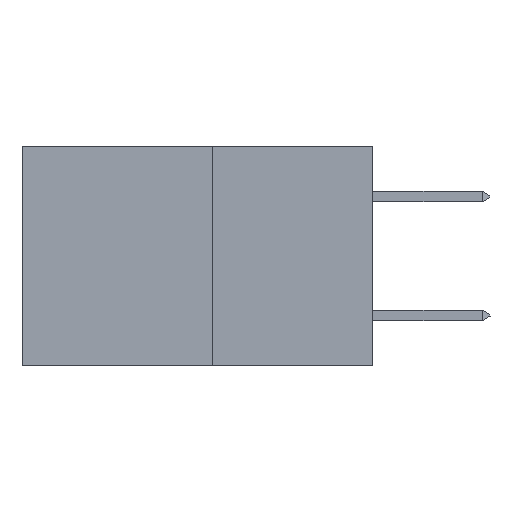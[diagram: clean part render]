
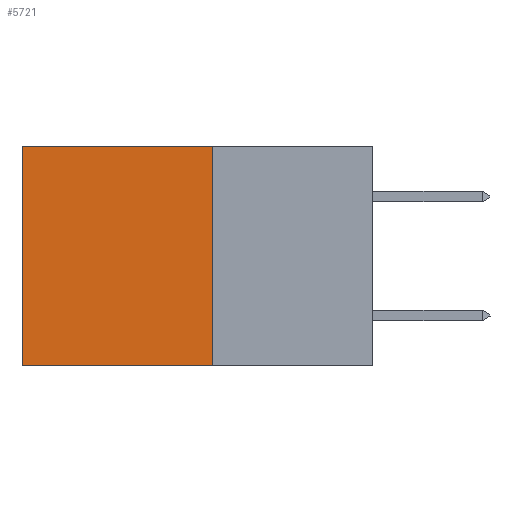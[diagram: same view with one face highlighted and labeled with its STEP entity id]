
A CAD part, left-side view. The second image highlights one B-rep face of the part: STEP entity #5721.
In plain terms, the highlighted planar face has unit normal (-1, 0, 0).
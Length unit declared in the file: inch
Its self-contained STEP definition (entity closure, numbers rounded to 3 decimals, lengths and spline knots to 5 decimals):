
#82 = AXIS2_PLACEMENT_3D ( 'NONE', #2713, #2704, #2680 ) ;
#160 = CARTESIAN_POINT ( 'NONE',  ( 0.277, 0.27, -0.37 ) ) ;
#296 = CARTESIAN_POINT ( 'NONE',  ( 0.277, 0.59, -0.37 ) ) ;
#460 = CARTESIAN_POINT ( 'NONE',  ( 0.277, 0.27, 0. ) ) ;
#487 = DIRECTION ( 'NONE',  ( 0., 1., 0. ) ) ;
#781 = EDGE_CURVE ( 'NONE', #8859, #3221, #3631, .T. ) ;
#1024 = DIRECTION ( 'NONE',  ( 0., 0., -1. ) ) ;
#1095 = VERTEX_POINT ( 'NONE', #5561 ) ;
#1116 = CARTESIAN_POINT ( 'NONE',  ( 0.277, 0.59, -0.37 ) ) ;
#2073 = LINE ( 'NONE', #460, #3802 ) ;
#2413 = CARTESIAN_POINT ( 'NONE',  ( 0.277, 0.27, -0.37 ) ) ;
#2680 = DIRECTION ( 'NONE',  ( 0., 0., -1. ) ) ;
#2704 = DIRECTION ( 'NONE',  ( 1., 0., 0. ) ) ;
#2713 = CARTESIAN_POINT ( 'NONE',  ( 0.277, 0.27, -0.37 ) ) ;
#2767 = PLANE ( 'NONE',  #82 ) ;
#3221 = VERTEX_POINT ( 'NONE', #2413 ) ;
#3456 = EDGE_CURVE ( 'NONE', #8859, #1095, #2073, .T. ) ;
#3483 = EDGE_CURVE ( 'NONE', #3221, #6343, #7754, .T. ) ;
#3631 = LINE ( 'NONE', #7511, #7600 ) ;
#3650 = ORIENTED_EDGE ( 'NONE', *, *, #3456, .T. ) ;
#3802 = VECTOR ( 'NONE', #7028, 39.37008 ) ;
#4950 = DIRECTION ( 'NONE',  ( 0., 0., -1. ) ) ;
#5561 = CARTESIAN_POINT ( 'NONE',  ( 0.277, 0.59, 0. ) ) ;
#5577 = EDGE_LOOP ( 'NONE', ( #9260, #6430, #9116, #3650 ) ) ;
#5721 = ADVANCED_FACE ( 'NONE', ( #6285 ), #2767, .F. ) ;
#5869 = VECTOR ( 'NONE', #487, 39.37008 ) ;
#6285 = FACE_OUTER_BOUND ( 'NONE', #5577, .T. ) ;
#6343 = VERTEX_POINT ( 'NONE', #296 ) ;
#6430 = ORIENTED_EDGE ( 'NONE', *, *, #3483, .F. ) ;
#7028 = DIRECTION ( 'NONE',  ( 0., 1., 0. ) ) ;
#7395 = EDGE_CURVE ( 'NONE', #1095, #6343, #7711, .T. ) ;
#7509 = VECTOR ( 'NONE', #1024, 39.37008 ) ;
#7511 = CARTESIAN_POINT ( 'NONE',  ( 0.277, 0.27, -0.37 ) ) ;
#7600 = VECTOR ( 'NONE', #4950, 39.37008 ) ;
#7711 = LINE ( 'NONE', #1116, #7509 ) ;
#7754 = LINE ( 'NONE', #160, #5869 ) ;
#8573 = CARTESIAN_POINT ( 'NONE',  ( 0.277, 0.27, 0. ) ) ;
#8859 = VERTEX_POINT ( 'NONE', #8573 ) ;
#9116 = ORIENTED_EDGE ( 'NONE', *, *, #781, .F. ) ;
#9260 = ORIENTED_EDGE ( 'NONE', *, *, #7395, .T. ) ;
